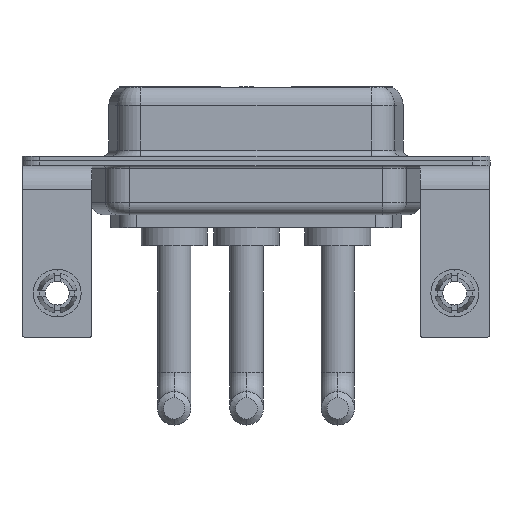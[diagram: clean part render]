
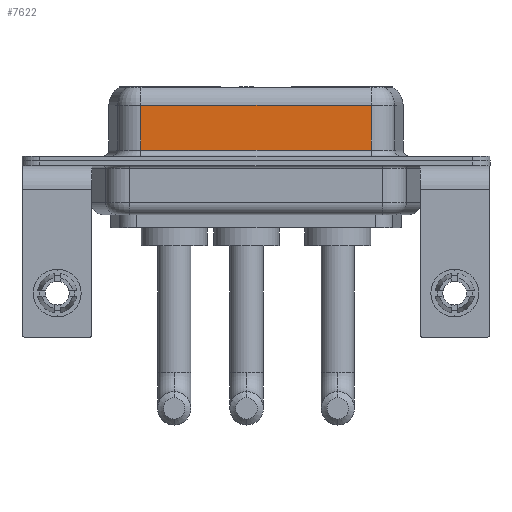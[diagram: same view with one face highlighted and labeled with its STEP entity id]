
A CAD part, front view. The second image highlights one B-rep face of the part: STEP entity #7622.
In plain terms, the highlighted planar face has unit normal (0, -1, 0).
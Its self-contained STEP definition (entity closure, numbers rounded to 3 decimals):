
#220 = VECTOR ( 'NONE', #7111, 1000. ) ;
#537 = EDGE_CURVE ( 'NONE', #14504, #8853, #1992, .T. ) ;
#909 = ORIENTED_EDGE ( 'NONE', *, *, #11594, .F. ) ;
#925 = CARTESIAN_POINT ( 'NONE',  ( 7.013, -3.95, 4.65 ) ) ;
#1323 = CARTESIAN_POINT ( 'NONE',  ( 26.287, -3.95, 4.65 ) ) ;
#1354 = ORIENTED_EDGE ( 'NONE', *, *, #537, .T. ) ;
#1992 = LINE ( 'NONE', #3705, #10241 ) ;
#2138 = CARTESIAN_POINT ( 'NONE',  ( 7.013, -3.95, 6.4 ) ) ;
#2291 = LINE ( 'NONE', #1323, #8316 ) ;
#2669 = PLANE ( 'NONE',  #11087 ) ;
#3072 = CARTESIAN_POINT ( 'NONE',  ( 7.013, -3.95, 0.9 ) ) ;
#3258 = CARTESIAN_POINT ( 'NONE',  ( 26.287, -3.95, 0.9 ) ) ;
#3705 = CARTESIAN_POINT ( 'NONE',  ( 26.287, -3.95, 0.9 ) ) ;
#4326 = DIRECTION ( 'NONE',  ( 0., 0., -1. ) ) ;
#4427 = EDGE_LOOP ( 'NONE', ( #909, #13088, #8795, #1354 ) ) ;
#6306 = DIRECTION ( 'NONE',  ( -1., 0., 0. ) ) ;
#7111 = DIRECTION ( 'NONE',  ( 0., 0., -1. ) ) ;
#7622 = ADVANCED_FACE ( 'NONE', ( #13792 ), #2669, .F. ) ;
#8316 = VECTOR ( 'NONE', #6306, 1000. ) ;
#8593 = CARTESIAN_POINT ( 'NONE',  ( 26.287, -3.95, 4.65 ) ) ;
#8795 = ORIENTED_EDGE ( 'NONE', *, *, #11495, .T. ) ;
#8853 = VERTEX_POINT ( 'NONE', #3258 ) ;
#10022 = CARTESIAN_POINT ( 'NONE',  ( 26.287, -3.95, 6.4 ) ) ;
#10241 = VECTOR ( 'NONE', #11973, 1000. ) ;
#11087 = AXIS2_PLACEMENT_3D ( 'NONE', #10022, #12640, #15016 ) ;
#11495 = EDGE_CURVE ( 'NONE', #12862, #14504, #14478, .T. ) ;
#11594 = EDGE_CURVE ( 'NONE', #11614, #8853, #15533, .T. ) ;
#11614 = VERTEX_POINT ( 'NONE', #8593 ) ;
#11718 = EDGE_CURVE ( 'NONE', #11614, #12862, #2291, .T. ) ;
#11973 = DIRECTION ( 'NONE',  ( 1., 0., 0. ) ) ;
#12640 = DIRECTION ( 'NONE',  ( 0., 1., 0. ) ) ;
#12862 = VERTEX_POINT ( 'NONE', #925 ) ;
#13088 = ORIENTED_EDGE ( 'NONE', *, *, #11718, .T. ) ;
#13792 = FACE_OUTER_BOUND ( 'NONE', #4427, .T. ) ;
#14478 = LINE ( 'NONE', #2138, #220 ) ;
#14504 = VERTEX_POINT ( 'NONE', #3072 ) ;
#15016 = DIRECTION ( 'NONE',  ( 0., 0., 1. ) ) ;
#15533 = LINE ( 'NONE', #15704, #15899 ) ;
#15704 = CARTESIAN_POINT ( 'NONE',  ( 26.287, -3.95, 6.4 ) ) ;
#15899 = VECTOR ( 'NONE', #4326, 1000. ) ;
